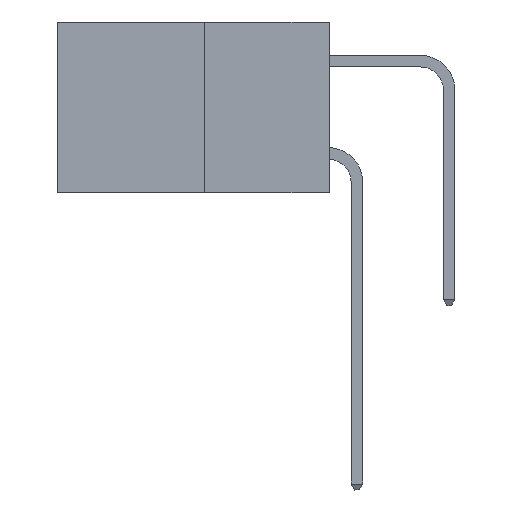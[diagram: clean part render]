
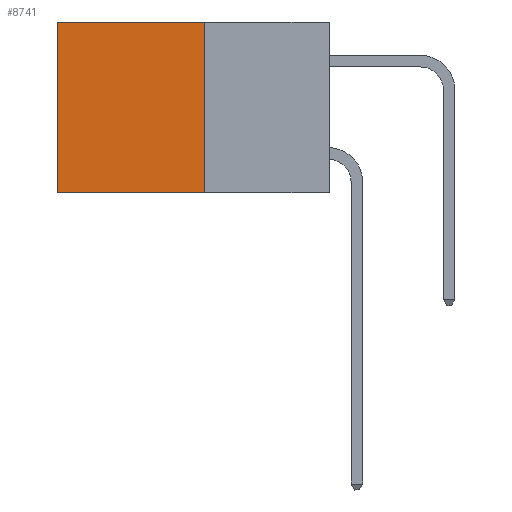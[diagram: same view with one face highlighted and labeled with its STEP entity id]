
A CAD part, left-side view. The second image highlights one B-rep face of the part: STEP entity #8741.
In plain terms, the highlighted planar face has unit normal (-1, 0, 0).
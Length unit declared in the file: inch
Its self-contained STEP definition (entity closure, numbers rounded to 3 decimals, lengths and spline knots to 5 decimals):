
#4 = CARTESIAN_POINT ( 'NONE',  ( 0.277, 0.27, -0.37 ) ) ;
#484 = CARTESIAN_POINT ( 'NONE',  ( 0.277, 0.59, -0.37 ) ) ;
#776 = VECTOR ( 'NONE', #5214, 39.37008 ) ;
#903 = ORIENTED_EDGE ( 'NONE', *, *, #7254, .F. ) ;
#1364 = ORIENTED_EDGE ( 'NONE', *, *, #9390, .T. ) ;
#1424 = CARTESIAN_POINT ( 'NONE',  ( 0.277, 0.27, 0. ) ) ;
#1804 = LINE ( 'NONE', #1424, #11490 ) ;
#1969 = CARTESIAN_POINT ( 'NONE',  ( 0.277, 0.27, -0.37 ) ) ;
#2296 = DIRECTION ( 'NONE',  ( 1., 0., 0. ) ) ;
#2300 = VERTEX_POINT ( 'NONE', #4 ) ;
#2528 = VERTEX_POINT ( 'NONE', #11829 ) ;
#2783 = CARTESIAN_POINT ( 'NONE',  ( 0.277, 0.59, 0. ) ) ;
#2929 = DIRECTION ( 'NONE',  ( 0., 0., -1. ) ) ;
#3452 = EDGE_CURVE ( 'NONE', #4314, #2528, #8436, .T. ) ;
#3759 = VECTOR ( 'NONE', #2929, 39.37008 ) ;
#4055 = LINE ( 'NONE', #1969, #3759 ) ;
#4314 = VERTEX_POINT ( 'NONE', #2783 ) ;
#4486 = FACE_OUTER_BOUND ( 'NONE', #11782, .T. ) ;
#4970 = CARTESIAN_POINT ( 'NONE',  ( 0.277, 0.27, -0.37 ) ) ;
#5070 = ORIENTED_EDGE ( 'NONE', *, *, #3452, .T. ) ;
#5100 = PLANE ( 'NONE',  #8971 ) ;
#5192 = DIRECTION ( 'NONE',  ( 0., 1., 0. ) ) ;
#5214 = DIRECTION ( 'NONE',  ( 0., 0., -1. ) ) ;
#5391 = VERTEX_POINT ( 'NONE', #10429 ) ;
#5894 = DIRECTION ( 'NONE',  ( 0., 1., 0. ) ) ;
#6398 = VECTOR ( 'NONE', #5894, 39.37008 ) ;
#7254 = EDGE_CURVE ( 'NONE', #2300, #2528, #8745, .T. ) ;
#7853 = ORIENTED_EDGE ( 'NONE', *, *, #8536, .F. ) ;
#8436 = LINE ( 'NONE', #484, #776 ) ;
#8536 = EDGE_CURVE ( 'NONE', #5391, #2300, #4055, .T. ) ;
#8688 = DIRECTION ( 'NONE',  ( 0., 0., -1. ) ) ;
#8741 = ADVANCED_FACE ( 'NONE', ( #4486 ), #5100, .F. ) ;
#8745 = LINE ( 'NONE', #4970, #6398 ) ;
#8971 = AXIS2_PLACEMENT_3D ( 'NONE', #9538, #2296, #8688 ) ;
#9390 = EDGE_CURVE ( 'NONE', #5391, #4314, #1804, .T. ) ;
#9538 = CARTESIAN_POINT ( 'NONE',  ( 0.277, 0.27, -0.37 ) ) ;
#10429 = CARTESIAN_POINT ( 'NONE',  ( 0.277, 0.27, 0. ) ) ;
#11490 = VECTOR ( 'NONE', #5192, 39.37008 ) ;
#11782 = EDGE_LOOP ( 'NONE', ( #5070, #903, #7853, #1364 ) ) ;
#11829 = CARTESIAN_POINT ( 'NONE',  ( 0.277, 0.59, -0.37 ) ) ;
